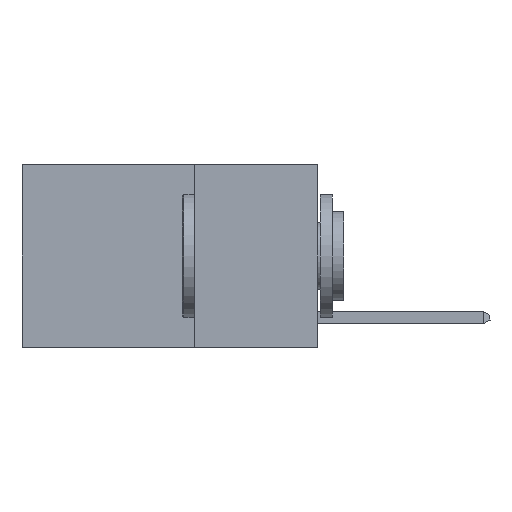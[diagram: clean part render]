
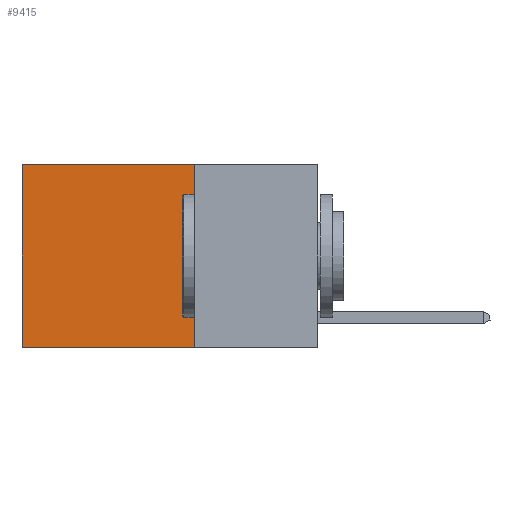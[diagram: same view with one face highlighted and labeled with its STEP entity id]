
A CAD part, left-side view. The second image highlights one B-rep face of the part: STEP entity #9415.
In plain terms, the highlighted planar face has unit normal (-1, 0, 0).
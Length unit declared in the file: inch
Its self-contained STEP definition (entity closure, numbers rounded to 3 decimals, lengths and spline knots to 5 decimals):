
#182 = LINE ( 'NONE', #10525, #8087 ) ;
#194 = DIRECTION ( 'NONE',  ( 0., 1., 0. ) ) ;
#409 = AXIS2_PLACEMENT_3D ( 'NONE', #14061, #8300, #18441 ) ;
#494 = CARTESIAN_POINT ( 'NONE',  ( 0.2625, 0.6, -0.37 ) ) ;
#1103 = VERTEX_POINT ( 'NONE', #494 ) ;
#1564 = FACE_OUTER_BOUND ( 'NONE', #7926, .T. ) ;
#1906 = CARTESIAN_POINT ( 'NONE',  ( 0.2625, 0.25, 0. ) ) ;
#2192 = CARTESIAN_POINT ( 'NONE',  ( 0.2625, 0.25, -0.37 ) ) ;
#2329 = PLANE ( 'NONE',  #409 ) ;
#2362 = CARTESIAN_POINT ( 'NONE',  ( 0.2625, 0.25, 0. ) ) ;
#3546 = VERTEX_POINT ( 'NONE', #7086 ) ;
#4120 = CARTESIAN_POINT ( 'NONE',  ( 0.2625, 0.25, -0.37 ) ) ;
#4473 = LINE ( 'NONE', #1906, #15668 ) ;
#5598 = DIRECTION ( 'NONE',  ( 0., 1., 0. ) ) ;
#6285 = ORIENTED_EDGE ( 'NONE', *, *, #7043, .F. ) ;
#6812 = DIRECTION ( 'NONE',  ( 0., 0., -1. ) ) ;
#7043 = EDGE_CURVE ( 'NONE', #9361, #1103, #12075, .T. ) ;
#7086 = CARTESIAN_POINT ( 'NONE',  ( 0.2625, 0.6, 0. ) ) ;
#7703 = ORIENTED_EDGE ( 'NONE', *, *, #15549, .F. ) ;
#7926 = EDGE_LOOP ( 'NONE', ( #14610, #6285, #7703, #17740 ) ) ;
#8087 = VECTOR ( 'NONE', #194, 39.37008 ) ;
#8300 = DIRECTION ( 'NONE',  ( 1., 0., 0. ) ) ;
#8916 = VERTEX_POINT ( 'NONE', #2362 ) ;
#9361 = VERTEX_POINT ( 'NONE', #2192 ) ;
#9415 = ADVANCED_FACE ( 'NONE', ( #1564 ), #2329, .F. ) ;
#10525 = CARTESIAN_POINT ( 'NONE',  ( 0.2625, 0.25, 0. ) ) ;
#10690 = EDGE_CURVE ( 'NONE', #3546, #1103, #15531, .T. ) ;
#12075 = LINE ( 'NONE', #4120, #15040 ) ;
#12179 = DIRECTION ( 'NONE',  ( 0., 0., -1. ) ) ;
#12621 = CARTESIAN_POINT ( 'NONE',  ( 0.2625, 0.6, 0. ) ) ;
#14061 = CARTESIAN_POINT ( 'NONE',  ( 0.2625, 0.25, 0. ) ) ;
#14610 = ORIENTED_EDGE ( 'NONE', *, *, #10690, .T. ) ;
#15040 = VECTOR ( 'NONE', #5598, 39.37008 ) ;
#15531 = LINE ( 'NONE', #12621, #18921 ) ;
#15549 = EDGE_CURVE ( 'NONE', #8916, #9361, #4473, .T. ) ;
#15668 = VECTOR ( 'NONE', #12179, 39.37008 ) ;
#17740 = ORIENTED_EDGE ( 'NONE', *, *, #17976, .T. ) ;
#17976 = EDGE_CURVE ( 'NONE', #8916, #3546, #182, .T. ) ;
#18441 = DIRECTION ( 'NONE',  ( 0., 0., -1. ) ) ;
#18921 = VECTOR ( 'NONE', #6812, 39.37008 ) ;
